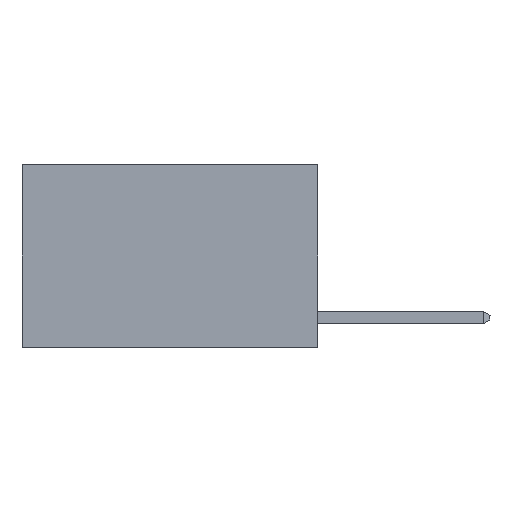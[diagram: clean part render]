
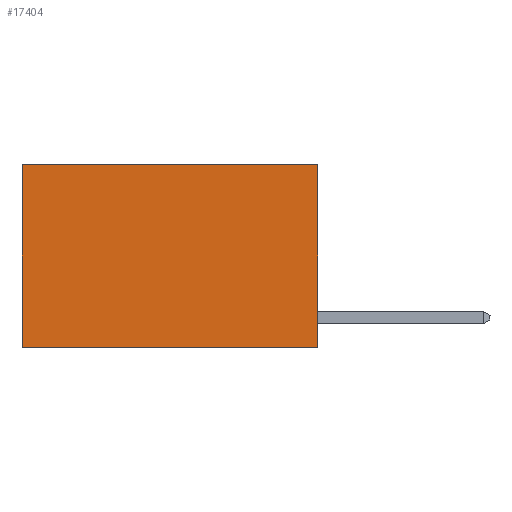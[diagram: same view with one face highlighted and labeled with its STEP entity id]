
A CAD part, left-side view. The second image highlights one B-rep face of the part: STEP entity #17404.
In plain terms, the highlighted planar face has unit normal (-1, 0, 0).
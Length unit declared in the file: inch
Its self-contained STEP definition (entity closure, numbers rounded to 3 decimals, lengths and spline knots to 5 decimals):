
#1937 = ORIENTED_EDGE ( 'NONE', *, *, #16354, .F. ) ;
#1996 = LINE ( 'NONE', #4433, #19087 ) ;
#2665 = VERTEX_POINT ( 'NONE', #12763 ) ;
#3480 = PLANE ( 'NONE',  #7879 ) ;
#4408 = ORIENTED_EDGE ( 'NONE', *, *, #4913, .T. ) ;
#4433 = CARTESIAN_POINT ( 'NONE',  ( 0.2625, 0., 0. ) ) ;
#4441 = DIRECTION ( 'NONE',  ( 0., 1., 0. ) ) ;
#4913 = EDGE_CURVE ( 'NONE', #2665, #9057, #6019, .T. ) ;
#6019 = LINE ( 'NONE', #22031, #11022 ) ;
#6580 = DIRECTION ( 'NONE',  ( 0., 1., 0. ) ) ;
#7730 = CARTESIAN_POINT ( 'NONE',  ( 0.2625, 0., 0. ) ) ;
#7879 = AXIS2_PLACEMENT_3D ( 'NONE', #7730, #22816, #9898 ) ;
#8000 = VERTEX_POINT ( 'NONE', #9829 ) ;
#9057 = VERTEX_POINT ( 'NONE', #21964 ) ;
#9829 = CARTESIAN_POINT ( 'NONE',  ( 0.2625, 0., 0. ) ) ;
#9898 = DIRECTION ( 'NONE',  ( 0., 0., -1. ) ) ;
#10787 = FACE_OUTER_BOUND ( 'NONE', #26676, .T. ) ;
#11022 = VECTOR ( 'NONE', #11276, 39.37008 ) ;
#11276 = DIRECTION ( 'NONE',  ( 0., 0., -1. ) ) ;
#11457 = ORIENTED_EDGE ( 'NONE', *, *, #19546, .T. ) ;
#12763 = CARTESIAN_POINT ( 'NONE',  ( 0.2625, 0.6, 0. ) ) ;
#12783 = EDGE_CURVE ( 'NONE', #8000, #20830, #19069, .T. ) ;
#16354 = EDGE_CURVE ( 'NONE', #20830, #9057, #27033, .T. ) ;
#17404 = ADVANCED_FACE ( 'NONE', ( #10787 ), #3480, .F. ) ;
#18370 = VECTOR ( 'NONE', #18570, 39.37008 ) ;
#18570 = DIRECTION ( 'NONE',  ( 0., 0., -1. ) ) ;
#19069 = LINE ( 'NONE', #25101, #18370 ) ;
#19087 = VECTOR ( 'NONE', #6580, 39.37008 ) ;
#19546 = EDGE_CURVE ( 'NONE', #8000, #2665, #1996, .T. ) ;
#20830 = VERTEX_POINT ( 'NONE', #21865 ) ;
#21319 = VECTOR ( 'NONE', #4441, 39.37008 ) ;
#21865 = CARTESIAN_POINT ( 'NONE',  ( 0.2625, 0., -0.37 ) ) ;
#21964 = CARTESIAN_POINT ( 'NONE',  ( 0.2625, 0.6, -0.37 ) ) ;
#22031 = CARTESIAN_POINT ( 'NONE',  ( 0.2625, 0.6, 0. ) ) ;
#22816 = DIRECTION ( 'NONE',  ( 1., 0., 0. ) ) ;
#23684 = CARTESIAN_POINT ( 'NONE',  ( 0.2625, 0., -0.37 ) ) ;
#24093 = ORIENTED_EDGE ( 'NONE', *, *, #12783, .F. ) ;
#25101 = CARTESIAN_POINT ( 'NONE',  ( 0.2625, 0., 0. ) ) ;
#26676 = EDGE_LOOP ( 'NONE', ( #4408, #1937, #24093, #11457 ) ) ;
#27033 = LINE ( 'NONE', #23684, #21319 ) ;
